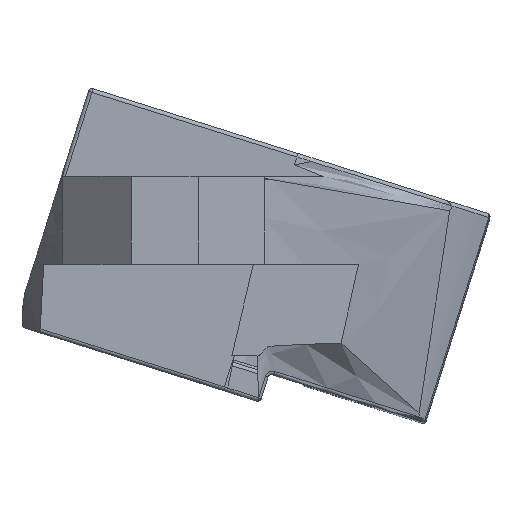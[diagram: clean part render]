
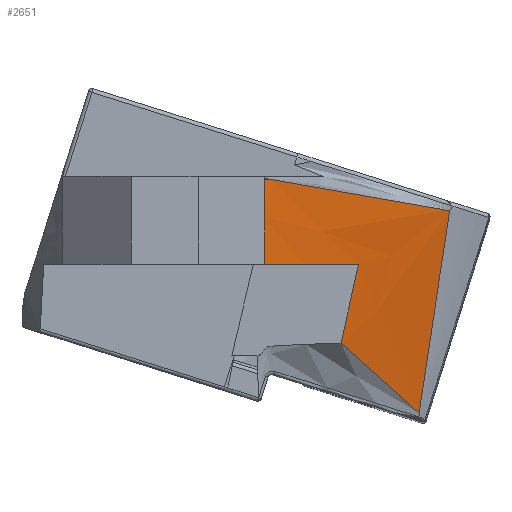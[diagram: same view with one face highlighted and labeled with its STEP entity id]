
A CAD part, top view. The second image highlights one B-rep face of the part: STEP entity #2651.
In plain terms, the highlighted free-form (B-spline) face has degree [3, 3] with [4, 4] control points.
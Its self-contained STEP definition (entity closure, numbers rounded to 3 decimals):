
#131=B_SPLINE_SURFACE_WITH_KNOTS('',3,3,((#9187,#9188,#9189,#9190),(#9191,
#9192,#9193,#9194),(#9195,#9196,#9197,#9198),(#9199,#9200,#9201,#9202)),
 .UNSPECIFIED.,.F.,.F.,.F.,(4,4),(4,4),(0.,1.),(0.037,
1.),.UNSPECIFIED.);
#337=B_SPLINE_CURVE_WITH_KNOTS('',3,(#8952,#8953,#8954,#8955,#8956,#8957,
#8958,#8959,#8960,#8961,#8962,#8963,#8964),.UNSPECIFIED.,.F.,.F.,(4,3,3,
3,4),(0.,0.225,0.333,0.519,0.705),
 .UNSPECIFIED.);
#345=B_SPLINE_CURVE_WITH_KNOTS('',3,(#9062,#9063,#9064,#9065,#9066,#9067),
 .UNSPECIFIED.,.F.,.F.,(4,2,4),(-0.047,0.,0.005),
 .UNSPECIFIED.);
#351=B_SPLINE_CURVE_WITH_KNOTS('',3,(#9155,#9156,#9157,#9158),
 .UNSPECIFIED.,.F.,.F.,(4,4),(-0.129,0.),.UNSPECIFIED.);
#353=B_SPLINE_CURVE_WITH_KNOTS('',3,(#9205,#9206,#9207,#9208),
 .UNSPECIFIED.,.F.,.F.,(4,4),(-0.275,0.),.UNSPECIFIED.);
#354=B_SPLINE_CURVE_WITH_KNOTS('',3,(#9212,#9213,#9214,#9215),
 .UNSPECIFIED.,.F.,.F.,(4,4),(-0.004,0.035),
 .UNSPECIFIED.);
#355=B_SPLINE_CURVE_WITH_KNOTS('',3,(#9216,#9217,#9218,#9219,#9220,#9221),
 .UNSPECIFIED.,.F.,.F.,(4,2,4),(-0.559,-0.338,-0.073),
 .UNSPECIFIED.);
#429=FACE_OUTER_BOUND('',#600,.T.);
#600=EDGE_LOOP('',(#2047,#2048,#2049,#2050,#2051,#2052,#2053,#2054,#2055,
#2056,#2057));
#759=LINE('',#9053,#945);
#760=LINE('',#9054,#946);
#763=LINE('',#9072,#949);
#769=LINE('',#9210,#955);
#770=LINE('',#9211,#956);
#945=VECTOR('',#3388,10.83);
#946=VECTOR('',#3389,10.83);
#949=VECTOR('',#3394,10.);
#955=VECTOR('',#3412,10.626);
#956=VECTOR('',#3413,10.626);
#1166=VERTEX_POINT('',#8928);
#1167=VERTEX_POINT('',#8951);
#1173=VERTEX_POINT('',#9047);
#1174=VERTEX_POINT('',#9052);
#1175=VERTEX_POINT('',#9060);
#1176=VERTEX_POINT('',#9061);
#1178=VERTEX_POINT('',#9070);
#1184=VERTEX_POINT('',#9154);
#1185=VERTEX_POINT('',#9203);
#1186=VERTEX_POINT('',#9204);
#1187=VERTEX_POINT('',#9209);
#1468=EDGE_CURVE('',#1166,#1167,#337,.T.);
#1477=EDGE_CURVE('',#1174,#1173,#759,.T.);
#1478=EDGE_CURVE('',#1166,#1174,#760,.T.);
#1480=EDGE_CURVE('',#1175,#1176,#345,.T.);
#1483=EDGE_CURVE('',#1176,#1178,#763,.T.);
#1495=EDGE_CURVE('',#1175,#1184,#351,.F.);
#1497=EDGE_CURVE('',#1185,#1186,#353,.T.);
#1498=EDGE_CURVE('',#1187,#1186,#769,.T.);
#1499=EDGE_CURVE('',#1167,#1187,#770,.T.);
#1500=EDGE_CURVE('',#1184,#1173,#354,.T.);
#1501=EDGE_CURVE('',#1178,#1185,#355,.T.);
#2047=ORIENTED_EDGE('',*,*,#1497,.T.);
#2048=ORIENTED_EDGE('',*,*,#1498,.F.);
#2049=ORIENTED_EDGE('',*,*,#1499,.F.);
#2050=ORIENTED_EDGE('',*,*,#1468,.F.);
#2051=ORIENTED_EDGE('',*,*,#1478,.T.);
#2052=ORIENTED_EDGE('',*,*,#1477,.T.);
#2053=ORIENTED_EDGE('',*,*,#1500,.F.);
#2054=ORIENTED_EDGE('',*,*,#1495,.F.);
#2055=ORIENTED_EDGE('',*,*,#1480,.T.);
#2056=ORIENTED_EDGE('',*,*,#1483,.T.);
#2057=ORIENTED_EDGE('',*,*,#1501,.T.);
#2651=ADVANCED_FACE('',(#429),#131,.F.);
#3388=DIRECTION('',(-0.742,0.128,0.658));
#3389=DIRECTION('',(-0.742,0.128,0.658));
#3394=DIRECTION('',(0.,-1.,0.));
#3412=DIRECTION('',(-0.552,0.495,0.671));
#3413=DIRECTION('',(-0.552,0.495,0.671));
#8928=CARTESIAN_POINT('',(61.348,-34.209,11.714));
#8951=CARTESIAN_POINT('',(60.3,-41.113,10.793));
#8952=CARTESIAN_POINT('Ctrl Pts',(61.348,-34.209,11.714));
#8953=CARTESIAN_POINT('Ctrl Pts',(61.244,-34.947,11.621));
#8954=CARTESIAN_POINT('Ctrl Pts',(61.138,-35.683,11.526));
#8955=CARTESIAN_POINT('Ctrl Pts',(61.029,-36.419,11.43));
#8956=CARTESIAN_POINT('Ctrl Pts',(60.977,-36.77,11.384));
#8957=CARTESIAN_POINT('Ctrl Pts',(60.925,-37.121,11.337));
#8958=CARTESIAN_POINT('Ctrl Pts',(60.872,-37.472,11.291));
#8959=CARTESIAN_POINT('Ctrl Pts',(60.78,-38.08,11.21));
#8960=CARTESIAN_POINT('Ctrl Pts',(60.687,-38.687,11.128));
#8961=CARTESIAN_POINT('Ctrl Pts',(60.591,-39.294,11.045));
#8962=CARTESIAN_POINT('Ctrl Pts',(60.496,-39.9,10.962));
#8963=CARTESIAN_POINT('Ctrl Pts',(60.399,-40.506,10.878));
#8964=CARTESIAN_POINT('Ctrl Pts',(60.3,-41.113,10.793));
#9047=CARTESIAN_POINT('',(55.294,-33.162,17.088));
#9052=CARTESIAN_POINT('',(61.239,-34.19,11.81));
#9053=CARTESIAN_POINT('',(62.682,-34.44,10.53));
#9054=CARTESIAN_POINT('',(62.682,-34.44,10.53));
#9060=CARTESIAN_POINT('',(55.004,-34.437,17.307));
#9061=CARTESIAN_POINT('',(54.65,-34.289,17.66));
#9062=CARTESIAN_POINT('Ctrl Pts',(55.004,-34.437,17.307));
#9063=CARTESIAN_POINT('Ctrl Pts',(54.896,-34.392,17.414));
#9064=CARTESIAN_POINT('Ctrl Pts',(54.789,-34.347,17.521));
#9065=CARTESIAN_POINT('Ctrl Pts',(54.671,-34.298,17.639));
#9066=CARTESIAN_POINT('Ctrl Pts',(54.661,-34.293,17.65));
#9067=CARTESIAN_POINT('Ctrl Pts',(54.65,-34.289,17.66));
#9070=CARTESIAN_POINT('',(54.649,-36.05,17.66));
#9072=CARTESIAN_POINT('',(54.65,-34.55,17.66));
#9154=CARTESIAN_POINT('',(55.007,-33.127,17.343));
#9155=CARTESIAN_POINT('Ctrl Pts',(55.007,-33.127,17.343));
#9156=CARTESIAN_POINT('Ctrl Pts',(55.006,-33.57,17.332));
#9157=CARTESIAN_POINT('Ctrl Pts',(55.005,-34.008,17.32));
#9158=CARTESIAN_POINT('Ctrl Pts',(55.004,-34.437,17.307));
#9187=CARTESIAN_POINT('Ctrl Pts',(62.385,-34.389,10.793));
#9188=CARTESIAN_POINT('Ctrl Pts',(59.807,-33.942,13.082));
#9189=CARTESIAN_POINT('Ctrl Pts',(57.228,-33.496,15.371));
#9190=CARTESIAN_POINT('Ctrl Pts',(54.65,-33.05,17.66));
#9191=CARTESIAN_POINT('Ctrl Pts',(61.69,-36.63,10.793));
#9192=CARTESIAN_POINT('Ctrl Pts',(59.343,-35.77,13.082));
#9193=CARTESIAN_POINT('Ctrl Pts',(56.997,-34.91,15.371));
#9194=CARTESIAN_POINT('Ctrl Pts',(54.65,-34.05,17.66));
#9195=CARTESIAN_POINT('Ctrl Pts',(60.995,-38.871,10.793));
#9196=CARTESIAN_POINT('Ctrl Pts',(58.88,-37.598,13.082));
#9197=CARTESIAN_POINT('Ctrl Pts',(56.765,-36.324,15.371));
#9198=CARTESIAN_POINT('Ctrl Pts',(54.65,-35.05,17.66));
#9199=CARTESIAN_POINT('Ctrl Pts',(60.3,-41.113,10.793));
#9200=CARTESIAN_POINT('Ctrl Pts',(58.417,-39.425,13.082));
#9201=CARTESIAN_POINT('Ctrl Pts',(56.533,-37.738,15.371));
#9202=CARTESIAN_POINT('Ctrl Pts',(54.65,-36.05,17.66));
#9203=CARTESIAN_POINT('',(58.236,-36.05,14.025));
#9204=CARTESIAN_POINT('',(57.641,-38.73,14.025));
#9205=CARTESIAN_POINT('Ctrl Pts',(58.236,-36.05,14.025));
#9206=CARTESIAN_POINT('Ctrl Pts',(58.038,-36.943,14.025));
#9207=CARTESIAN_POINT('Ctrl Pts',(57.839,-37.837,14.025));
#9208=CARTESIAN_POINT('Ctrl Pts',(57.641,-38.73,14.025));
#9209=CARTESIAN_POINT('',(60.246,-41.064,10.859));
#9210=CARTESIAN_POINT('',(60.517,-41.307,10.53));
#9211=CARTESIAN_POINT('',(60.517,-41.307,10.53));
#9212=CARTESIAN_POINT('Ctrl Pts',(55.007,-33.127,17.343));
#9213=CARTESIAN_POINT('Ctrl Pts',(55.102,-33.14,17.258));
#9214=CARTESIAN_POINT('Ctrl Pts',(55.198,-33.151,17.173));
#9215=CARTESIAN_POINT('Ctrl Pts',(55.294,-33.162,17.088));
#9216=CARTESIAN_POINT('Ctrl Pts',(54.65,-36.05,17.66));
#9217=CARTESIAN_POINT('Ctrl Pts',(55.13,-36.05,17.077));
#9218=CARTESIAN_POINT('Ctrl Pts',(55.707,-36.05,16.469));
#9219=CARTESIAN_POINT('Ctrl Pts',(56.864,-36.05,15.307));
#9220=CARTESIAN_POINT('Ctrl Pts',(57.562,-36.05,14.646));
#9221=CARTESIAN_POINT('Ctrl Pts',(58.236,-36.05,14.025));
